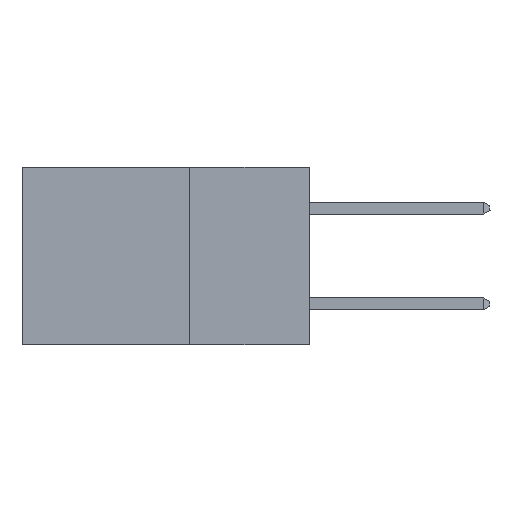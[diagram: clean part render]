
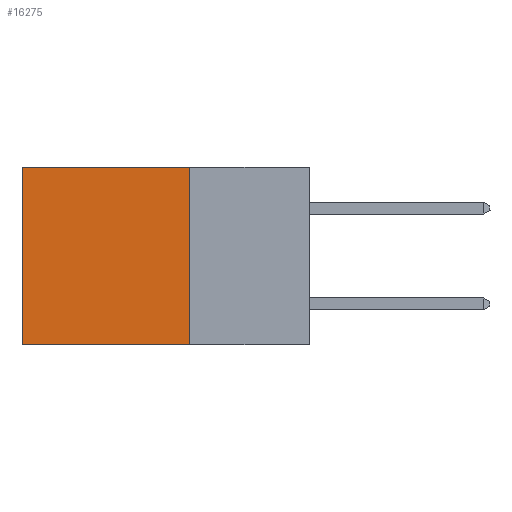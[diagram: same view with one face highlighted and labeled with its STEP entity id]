
A CAD part, left-side view. The second image highlights one B-rep face of the part: STEP entity #16275.
In plain terms, the highlighted planar face has unit normal (-1, 0, 0).
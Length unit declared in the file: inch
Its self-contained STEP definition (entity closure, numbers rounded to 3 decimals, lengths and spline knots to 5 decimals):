
#185 = DIRECTION ( 'NONE',  ( 0., 0., -1. ) ) ;
#487 = DIRECTION ( 'NONE',  ( 1., 0., 0. ) ) ;
#1296 = CARTESIAN_POINT ( 'NONE',  ( 0.2875, 0.25, 0. ) ) ;
#3244 = FACE_OUTER_BOUND ( 'NONE', #13923, .T. ) ;
#3388 = VECTOR ( 'NONE', #21596, 39.37008 ) ;
#3476 = VECTOR ( 'NONE', #20586, 39.37008 ) ;
#3604 = CARTESIAN_POINT ( 'NONE',  ( 0.2875, 0.25, -0.37 ) ) ;
#4759 = EDGE_CURVE ( 'NONE', #11339, #11419, #5366, .T. ) ;
#5335 = VERTEX_POINT ( 'NONE', #7214 ) ;
#5366 = LINE ( 'NONE', #13489, #3388 ) ;
#6668 = AXIS2_PLACEMENT_3D ( 'NONE', #24821, #487, #10474 ) ;
#7214 = CARTESIAN_POINT ( 'NONE',  ( 0.2875, 0.25, -0.37 ) ) ;
#7395 = EDGE_CURVE ( 'NONE', #19407, #11339, #12490, .T. ) ;
#7754 = EDGE_CURVE ( 'NONE', #19407, #5335, #18424, .T. ) ;
#7765 = ORIENTED_EDGE ( 'NONE', *, *, #7395, .T. ) ;
#8291 = CARTESIAN_POINT ( 'NONE',  ( 0.2875, 0.6, 0. ) ) ;
#9764 = EDGE_CURVE ( 'NONE', #5335, #11419, #21832, .T. ) ;
#10376 = CARTESIAN_POINT ( 'NONE',  ( 0.2875, 0.25, 0. ) ) ;
#10474 = DIRECTION ( 'NONE',  ( 0., 0., -1. ) ) ;
#11339 = VERTEX_POINT ( 'NONE', #8291 ) ;
#11419 = VERTEX_POINT ( 'NONE', #15305 ) ;
#11753 = ORIENTED_EDGE ( 'NONE', *, *, #4759, .T. ) ;
#11815 = ORIENTED_EDGE ( 'NONE', *, *, #7754, .F. ) ;
#12490 = LINE ( 'NONE', #24839, #3476 ) ;
#13218 = VECTOR ( 'NONE', #185, 39.37008 ) ;
#13489 = CARTESIAN_POINT ( 'NONE',  ( 0.2875, 0.6, 0. ) ) ;
#13923 = EDGE_LOOP ( 'NONE', ( #11753, #26120, #11815, #7765 ) ) ;
#15305 = CARTESIAN_POINT ( 'NONE',  ( 0.2875, 0.6, -0.37 ) ) ;
#16275 = ADVANCED_FACE ( 'NONE', ( #3244 ), #19467, .F. ) ;
#18424 = LINE ( 'NONE', #1296, #13218 ) ;
#18815 = VECTOR ( 'NONE', #26198, 39.37008 ) ;
#19407 = VERTEX_POINT ( 'NONE', #10376 ) ;
#19467 = PLANE ( 'NONE',  #6668 ) ;
#20586 = DIRECTION ( 'NONE',  ( 0., 1., 0. ) ) ;
#21596 = DIRECTION ( 'NONE',  ( 0., 0., -1. ) ) ;
#21832 = LINE ( 'NONE', #3604, #18815 ) ;
#24821 = CARTESIAN_POINT ( 'NONE',  ( 0.2875, 0.25, 0. ) ) ;
#24839 = CARTESIAN_POINT ( 'NONE',  ( 0.2875, 0.25, 0. ) ) ;
#26120 = ORIENTED_EDGE ( 'NONE', *, *, #9764, .F. ) ;
#26198 = DIRECTION ( 'NONE',  ( 0., 1., 0. ) ) ;
